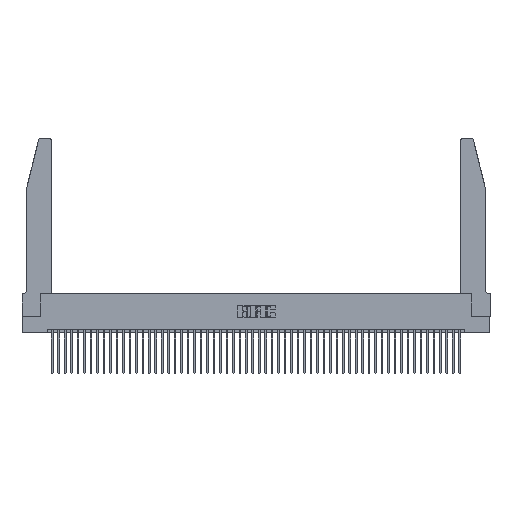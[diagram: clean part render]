
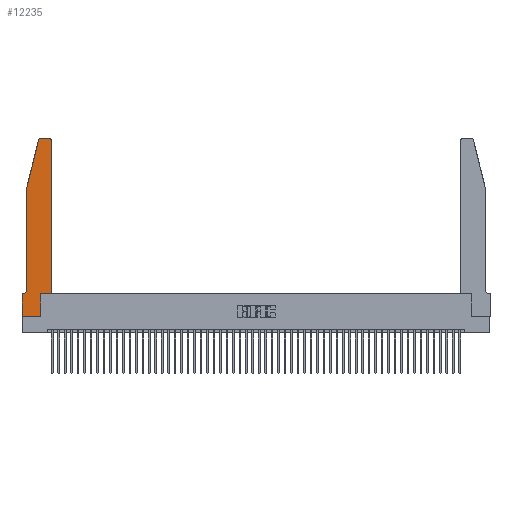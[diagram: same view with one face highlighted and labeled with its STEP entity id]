
A CAD part, top view. The second image highlights one B-rep face of the part: STEP entity #12235.
In plain terms, the highlighted planar face has unit normal (0, 0, 1).
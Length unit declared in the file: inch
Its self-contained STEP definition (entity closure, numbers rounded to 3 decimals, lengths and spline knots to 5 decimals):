
#348 = DIRECTION ( 'NONE',  ( 1., 0., 0. ) ) ;
#557 = VECTOR ( 'NONE', #19091, 39.37008 ) ;
#708 = DIRECTION ( 'NONE',  ( 0., 1., 0. ) ) ;
#781 = LINE ( 'NONE', #30996, #10422 ) ;
#1334 = VERTEX_POINT ( 'NONE', #34728 ) ;
#1855 = DIRECTION ( 'NONE',  ( 0., 0., 1. ) ) ;
#2033 = EDGE_LOOP ( 'NONE', ( #43110, #47143, #10838, #38317, #6643, #43280, #40433, #43080, #50026, #33131, #31656, #41091 ) ) ;
#2388 = CARTESIAN_POINT ( 'NONE',  ( 0.284, 2.72, 0.37 ) ) ;
#3135 = DIRECTION ( 'NONE',  ( 0., 1., 0. ) ) ;
#3728 = EDGE_CURVE ( 'NONE', #21650, #42767, #6532, .T. ) ;
#4013 = FACE_OUTER_BOUND ( 'NONE', #2033, .T. ) ;
#5352 = AXIS2_PLACEMENT_3D ( 'NONE', #26086, #1855, #30135 ) ;
#5961 = EDGE_CURVE ( 'NONE', #29003, #13951, #32819, .T. ) ;
#6526 = DIRECTION ( 'NONE',  ( 1., 0., 0. ) ) ;
#6532 = LINE ( 'NONE', #45723, #46696 ) ;
#6643 = ORIENTED_EDGE ( 'NONE', *, *, #22041, .T. ) ;
#7548 = AXIS2_PLACEMENT_3D ( 'NONE', #2388, #30659, #6526 ) ;
#7754 = CARTESIAN_POINT ( 'NONE',  ( 0.4505, 2.72, 0.37 ) ) ;
#10422 = VECTOR ( 'NONE', #10978, 39.37008 ) ;
#10676 = VECTOR ( 'NONE', #43450, 39.37008 ) ;
#10838 = ORIENTED_EDGE ( 'NONE', *, *, #27744, .T. ) ;
#10936 = CARTESIAN_POINT ( 'NONE',  ( 0.0755, 0.35, 0.37 ) ) ;
#10978 = DIRECTION ( 'NONE',  ( 1., 0., 0. ) ) ;
#11152 = CARTESIAN_POINT ( 'NONE',  ( 0.4205, 2.75, 0.37 ) ) ;
#11513 = CARTESIAN_POINT ( 'NONE',  ( 0., 0., 0.37 ) ) ;
#12167 = LINE ( 'NONE', #42307, #39136 ) ;
#12235 = ADVANCED_FACE ( 'NONE', ( #4013 ), #20587, .T. ) ;
#13951 = VERTEX_POINT ( 'NONE', #39539 ) ;
#14345 = DIRECTION ( 'NONE',  ( 0., -1., 0. ) ) ;
#15002 = DIRECTION ( 'NONE',  ( -1., 0., 0. ) ) ;
#15646 = CARTESIAN_POINT ( 'NONE',  ( 0., 0., 0.37 ) ) ;
#16919 = EDGE_CURVE ( 'NONE', #42767, #28306, #40744, .T. ) ;
#17321 = VERTEX_POINT ( 'NONE', #11513 ) ;
#17734 = VECTOR ( 'NONE', #15002, 39.37008 ) ;
#19091 = DIRECTION ( 'NONE',  ( 1., 0., 0. ) ) ;
#20587 = PLANE ( 'NONE',  #37003 ) ;
#20964 = EDGE_CURVE ( 'NONE', #22541, #29003, #50980, .T. ) ;
#21612 = DIRECTION ( 'NONE',  ( 0., 0., -1. ) ) ;
#21650 = VERTEX_POINT ( 'NONE', #11152 ) ;
#21743 = VERTEX_POINT ( 'NONE', #7754 ) ;
#21768 = DIRECTION ( 'NONE',  ( -1., 0., 0. ) ) ;
#22041 = EDGE_CURVE ( 'NONE', #48996, #1334, #34780, .T. ) ;
#22541 = VERTEX_POINT ( 'NONE', #24406 ) ;
#24406 = CARTESIAN_POINT ( 'NONE',  ( 0.2865, 0., 0.37 ) ) ;
#24642 = DIRECTION ( 'NONE',  ( 0., 0., 1. ) ) ;
#26086 = CARTESIAN_POINT ( 'NONE',  ( 0.4205, 2.72, 0.37 ) ) ;
#26984 = CARTESIAN_POINT ( 'NONE',  ( 0.4505, 0.35, 0.37 ) ) ;
#27354 = CARTESIAN_POINT ( 'NONE',  ( 0.2865, 0.35, 0.37 ) ) ;
#27744 = EDGE_CURVE ( 'NONE', #28306, #29318, #33925, .T. ) ;
#28306 = VERTEX_POINT ( 'NONE', #51263 ) ;
#28487 = CARTESIAN_POINT ( 'NONE',  ( 0.0755, 0.42, 0.37 ) ) ;
#28593 = AXIS2_PLACEMENT_3D ( 'NONE', #45578, #21612, #49556 ) ;
#29003 = VERTEX_POINT ( 'NONE', #31528 ) ;
#29318 = VERTEX_POINT ( 'NONE', #43348 ) ;
#30135 = DIRECTION ( 'NONE',  ( 1., 0., 0. ) ) ;
#30659 = DIRECTION ( 'NONE',  ( 0., 0., 1. ) ) ;
#30996 = CARTESIAN_POINT ( 'NONE',  ( 0., 0., 0.37 ) ) ;
#31528 = CARTESIAN_POINT ( 'NONE',  ( 0.2865, 0.35, 0.37 ) ) ;
#31656 = ORIENTED_EDGE ( 'NONE', *, *, #34444, .T. ) ;
#32034 = LINE ( 'NONE', #15646, #10676 ) ;
#32067 = EDGE_CURVE ( 'NONE', #29318, #48996, #12167, .T. ) ;
#32819 = LINE ( 'NONE', #26984, #557 ) ;
#33131 = ORIENTED_EDGE ( 'NONE', *, *, #5961, .T. ) ;
#33925 = LINE ( 'NONE', #43853, #43288 ) ;
#34444 = EDGE_CURVE ( 'NONE', #13951, #21743, #51293, .T. ) ;
#34728 = CARTESIAN_POINT ( 'NONE',  ( 0.0055, 0.35, 0.37 ) ) ;
#34780 = CIRCLE ( 'NONE', #28593, 0.07 ) ;
#36426 = CARTESIAN_POINT ( 'NONE',  ( 0.284, 2.75, 0.37 ) ) ;
#36896 = CARTESIAN_POINT ( 'NONE',  ( 0.4505, 0.35, 0.37 ) ) ;
#37003 = AXIS2_PLACEMENT_3D ( 'NONE', #48549, #24642, #348 ) ;
#38317 = ORIENTED_EDGE ( 'NONE', *, *, #32067, .T. ) ;
#38808 = EDGE_CURVE ( 'NONE', #1334, #46998, #39084, .T. ) ;
#39084 = LINE ( 'NONE', #10936, #17734 ) ;
#39136 = VECTOR ( 'NONE', #14345, 39.37008 ) ;
#39539 = CARTESIAN_POINT ( 'NONE',  ( 0.4505, 0.35, 0.37 ) ) ;
#39864 = DIRECTION ( 'NONE',  ( -0.239, -0.971, 0. ) ) ;
#40433 = ORIENTED_EDGE ( 'NONE', *, *, #51534, .T. ) ;
#40723 = VECTOR ( 'NONE', #708, 39.37008 ) ;
#40744 = CIRCLE ( 'NONE', #7548, 0.03 ) ;
#41091 = ORIENTED_EDGE ( 'NONE', *, *, #51955, .T. ) ;
#41649 = VECTOR ( 'NONE', #3135, 39.37008 ) ;
#41741 = CARTESIAN_POINT ( 'NONE',  ( 0., 0.35, 0.37 ) ) ;
#42307 = CARTESIAN_POINT ( 'NONE',  ( 0.0755, 2., 0.37 ) ) ;
#42767 = VERTEX_POINT ( 'NONE', #36426 ) ;
#43080 = ORIENTED_EDGE ( 'NONE', *, *, #43208, .T. ) ;
#43110 = ORIENTED_EDGE ( 'NONE', *, *, #3728, .T. ) ;
#43208 = EDGE_CURVE ( 'NONE', #17321, #22541, #781, .T. ) ;
#43280 = ORIENTED_EDGE ( 'NONE', *, *, #38808, .T. ) ;
#43288 = VECTOR ( 'NONE', #39864, 39.37008 ) ;
#43348 = CARTESIAN_POINT ( 'NONE',  ( 0.0755, 2., 0.37 ) ) ;
#43450 = DIRECTION ( 'NONE',  ( 0., -1., 0. ) ) ;
#43853 = CARTESIAN_POINT ( 'NONE',  ( 0.0755, 2., 0.37 ) ) ;
#45578 = CARTESIAN_POINT ( 'NONE',  ( 0.0055, 0.42, 0.37 ) ) ;
#45723 = CARTESIAN_POINT ( 'NONE',  ( 0.2605, 2.75, 0.37 ) ) ;
#46696 = VECTOR ( 'NONE', #21768, 39.37008 ) ;
#46998 = VERTEX_POINT ( 'NONE', #41741 ) ;
#47143 = ORIENTED_EDGE ( 'NONE', *, *, #16919, .T. ) ;
#47583 = CIRCLE ( 'NONE', #5352, 0.03 ) ;
#48549 = CARTESIAN_POINT ( 'NONE',  ( 0., 0.35, 0.37 ) ) ;
#48996 = VERTEX_POINT ( 'NONE', #28487 ) ;
#49556 = DIRECTION ( 'NONE',  ( -1., 0., 0. ) ) ;
#50026 = ORIENTED_EDGE ( 'NONE', *, *, #20964, .T. ) ;
#50980 = LINE ( 'NONE', #27354, #41649 ) ;
#51263 = CARTESIAN_POINT ( 'NONE',  ( 0.25487, 2.72718, 0.37 ) ) ;
#51293 = LINE ( 'NONE', #36896, #40723 ) ;
#51534 = EDGE_CURVE ( 'NONE', #46998, #17321, #32034, .T. ) ;
#51955 = EDGE_CURVE ( 'NONE', #21743, #21650, #47583, .T. ) ;
